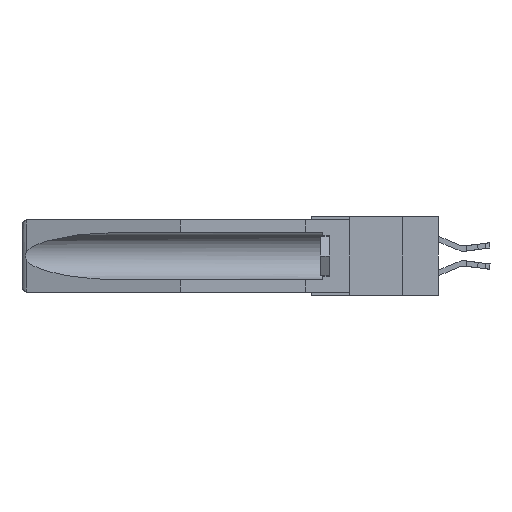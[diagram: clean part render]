
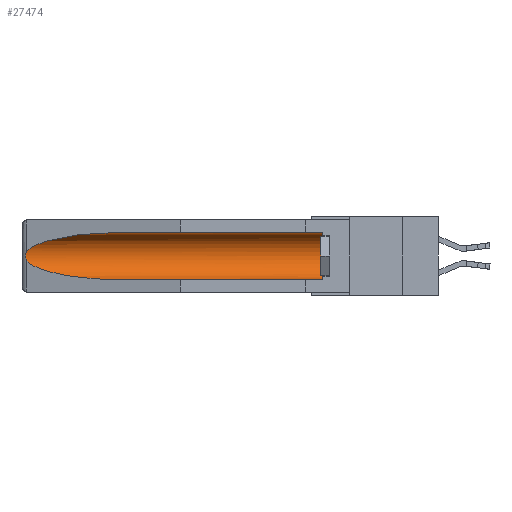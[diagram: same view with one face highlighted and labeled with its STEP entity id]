
A CAD part, left-side view. The second image highlights one B-rep face of the part: STEP entity #27474.
In plain terms, the highlighted cylindrical face has radius 2.857 mm (diameter 5.715 mm), a partial arc.
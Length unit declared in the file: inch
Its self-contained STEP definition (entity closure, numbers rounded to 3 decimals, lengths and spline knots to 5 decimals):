
#77 =( BOUNDED_CURVE ( )  B_SPLINE_CURVE ( 3, ( #12891, #6244, #21925, #4685 ),
 .UNSPECIFIED., .F., .F. ) 
 B_SPLINE_CURVE_WITH_KNOTS ( ( 4, 4 ),
 ( 4.71239, 6.08839 ),
 .UNSPECIFIED. ) 
 CURVE ( )  GEOMETRIC_REPRESENTATION_ITEM ( )  RATIONAL_B_SPLINE_CURVE ( ( 1., 0.848, 0.848, 1. ) ) 
 REPRESENTATION_ITEM ( '' )  );
#88 = DIRECTION ( 'NONE',  ( 0., 0., 1. ) ) ;
#1571 = AXIS2_PLACEMENT_3D ( 'NONE', #4454, #20198, #88 ) ;
#1713 = ORIENTED_EDGE ( 'NONE', *, *, #17690, .T. ) ;
#1811 = CARTESIAN_POINT ( 'NONE',  ( 0.155, -0.30754, -0.284 ) ) ;
#1880 = CARTESIAN_POINT ( 'NONE',  ( 0.155, 1.07973, -0.059 ) ) ;
#2412 = CARTESIAN_POINT ( 'NONE',  ( 0.155, 0.126, -0.059 ) ) ;
#3210 = EDGE_CURVE ( 'NONE', #25056, #5825, #10138, .T. ) ;
#3595 = CARTESIAN_POINT ( 'NONE',  ( 0.21114, 1.30732, -0.284 ) ) ;
#4101 = CARTESIAN_POINT ( 'NONE',  ( 0.2673, 1.53269, -0.17917 ) ) ;
#4313 = CARTESIAN_POINT ( 'NONE',  ( 0.26537, 1.52718, -0.14972 ) ) ;
#4454 = CARTESIAN_POINT ( 'NONE',  ( 0.155, 0.126, -0.1715 ) ) ;
#4509 = CARTESIAN_POINT ( 'NONE',  ( 0.2673, 1.5327, -0.16383 ) ) ;
#4685 = CARTESIAN_POINT ( 'NONE',  ( 0.26537, 1.52718, -0.14972 ) ) ;
#5825 = VERTEX_POINT ( 'NONE', #11480 ) ;
#6056 = VERTEX_POINT ( 'NONE', #1880 ) ;
#6244 = CARTESIAN_POINT ( 'NONE',  ( 0.21114, 1.30732, -0.059 ) ) ;
#6454 = CARTESIAN_POINT ( 'NONE',  ( 0.2675, 1.53308, -0.16763 ) ) ;
#7979 = LINE ( 'NONE', #1811, #28303 ) ;
#8092 = CARTESIAN_POINT ( 'NONE',  ( 0.155, 1.07973, -0.284 ) ) ;
#8783 = CARTESIAN_POINT ( 'NONE',  ( 0.2675, 1.53308, -0.17534 ) ) ;
#9593 = CARTESIAN_POINT ( 'NONE',  ( 0.155, -0.30754, -0.1715 ) ) ;
#10004 = FACE_OUTER_BOUND ( 'NONE', #23012, .T. ) ;
#10138 = B_SPLINE_CURVE_WITH_KNOTS ( 'NONE', 3,
 ( #4313, #28963, #17602, #4509, #6454, #8783, #4101, #24477, #26804, #13397 ),
 .UNSPECIFIED., .F., .F.,
 ( 4, 2, 2, 2, 4 ),
 ( 0., 0.00029, 0.00058, 0.00087, 0.00117 ),
 .UNSPECIFIED. ) ;
#11367 = EDGE_CURVE ( 'NONE', #5825, #17162, #23293, .T. ) ;
#11480 = CARTESIAN_POINT ( 'NONE',  ( 0.26537, 1.52718, -0.19328 ) ) ;
#12318 = CARTESIAN_POINT ( 'NONE',  ( 0.25451, 1.48313, -0.24835 ) ) ;
#12891 = CARTESIAN_POINT ( 'NONE',  ( 0.155, 1.07973, -0.059 ) ) ;
#13014 = LINE ( 'NONE', #15821, #18645 ) ;
#13397 = CARTESIAN_POINT ( 'NONE',  ( 0.26537, 1.52718, -0.19328 ) ) ;
#13812 = DIRECTION ( 'NONE',  ( 0., 1., 0. ) ) ;
#14763 = CARTESIAN_POINT ( 'NONE',  ( 0.26537, 1.52718, -0.19328 ) ) ;
#15821 = CARTESIAN_POINT ( 'NONE',  ( 0.155, -0.30754, -0.059 ) ) ;
#16038 = DIRECTION ( 'NONE',  ( 0., 0., 1. ) ) ;
#16292 = CYLINDRICAL_SURFACE ( 'NONE', #17232, 0.1125 ) ;
#16389 = VERTEX_POINT ( 'NONE', #18922 ) ;
#16802 = CIRCLE ( 'NONE', #1571, 0.1125 ) ;
#17162 = VERTEX_POINT ( 'NONE', #21086 ) ;
#17232 = AXIS2_PLACEMENT_3D ( 'NONE', #9593, #13812, #16038 ) ;
#17602 = CARTESIAN_POINT ( 'NONE',  ( 0.26654, 1.53092, -0.15636 ) ) ;
#17690 = EDGE_CURVE ( 'NONE', #6056, #25056, #77, .T. ) ;
#18096 = DIRECTION ( 'NONE',  ( 0., 1., 0. ) ) ;
#18645 = VECTOR ( 'NONE', #18096, 39.37008 ) ;
#18922 = CARTESIAN_POINT ( 'NONE',  ( 0.155, 0.126, -0.284 ) ) ;
#19497 = EDGE_CURVE ( 'NONE', #22053, #6056, #13014, .T. ) ;
#20198 = DIRECTION ( 'NONE',  ( 0., -1., 0. ) ) ;
#20223 = CARTESIAN_POINT ( 'NONE',  ( 0.26537, 1.52718, -0.14972 ) ) ;
#21086 = CARTESIAN_POINT ( 'NONE',  ( 0.155, 1.07973, -0.284 ) ) ;
#21925 = CARTESIAN_POINT ( 'NONE',  ( 0.25451, 1.48313, -0.09465 ) ) ;
#22053 = VERTEX_POINT ( 'NONE', #2412 ) ;
#22191 = EDGE_CURVE ( 'NONE', #16389, #22053, #16802, .T. ) ;
#23012 = EDGE_LOOP ( 'NONE', ( #1713, #25756, #26392, #27298, #25340, #24660 ) ) ;
#23293 =( BOUNDED_CURVE ( )  B_SPLINE_CURVE ( 3, ( #14763, #12318, #3595, #8092 ),
 .UNSPECIFIED., .F., .F. ) 
 B_SPLINE_CURVE_WITH_KNOTS ( ( 4, 4 ),
 ( 0.1948, 1.5708 ),
 .UNSPECIFIED. ) 
 CURVE ( )  GEOMETRIC_REPRESENTATION_ITEM ( )  RATIONAL_B_SPLINE_CURVE ( ( 1., 0.848, 0.848, 1. ) ) 
 REPRESENTATION_ITEM ( '' )  );
#24477 = CARTESIAN_POINT ( 'NONE',  ( 0.26655, 1.53094, -0.18657 ) ) ;
#24660 = ORIENTED_EDGE ( 'NONE', *, *, #19497, .T. ) ;
#25056 = VERTEX_POINT ( 'NONE', #20223 ) ;
#25340 = ORIENTED_EDGE ( 'NONE', *, *, #22191, .T. ) ;
#25756 = ORIENTED_EDGE ( 'NONE', *, *, #3210, .T. ) ;
#26210 = EDGE_CURVE ( 'NONE', #16389, #17162, #7979, .T. ) ;
#26392 = ORIENTED_EDGE ( 'NONE', *, *, #11367, .T. ) ;
#26804 = CARTESIAN_POINT ( 'NONE',  ( 0.26597, 1.5296, -0.19026 ) ) ;
#26883 = DIRECTION ( 'NONE',  ( 0., 1., 0. ) ) ;
#27298 = ORIENTED_EDGE ( 'NONE', *, *, #26210, .F. ) ;
#27474 = ADVANCED_FACE ( 'NONE', ( #10004 ), #16292, .F. ) ;
#28303 = VECTOR ( 'NONE', #26883, 39.37008 ) ;
#28963 = CARTESIAN_POINT ( 'NONE',  ( 0.26597, 1.52961, -0.15275 ) ) ;
